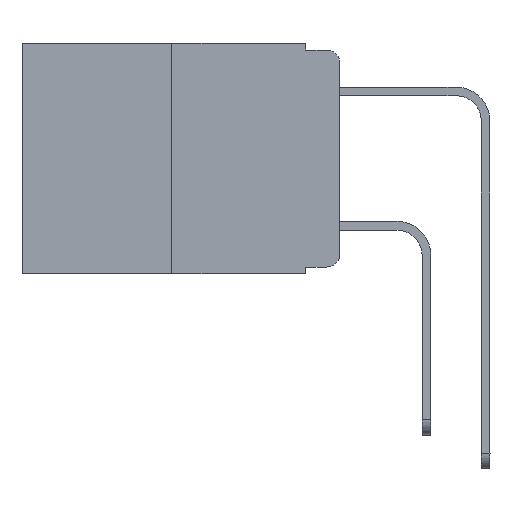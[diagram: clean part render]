
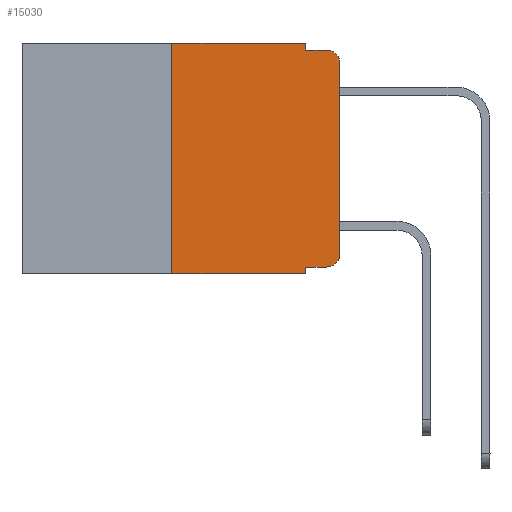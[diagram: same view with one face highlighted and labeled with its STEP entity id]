
A CAD part, left-side view. The second image highlights one B-rep face of the part: STEP entity #15030.
In plain terms, the highlighted planar face has unit normal (-1, 0, 0).
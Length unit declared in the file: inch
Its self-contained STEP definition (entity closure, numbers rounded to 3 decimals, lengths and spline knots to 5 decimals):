
#207 = EDGE_CURVE ( 'NONE', #6247, #10299, #6073, .T. ) ;
#486 = CARTESIAN_POINT ( 'NONE',  ( 0., 0., -0.313 ) ) ;
#516 = ORIENTED_EDGE ( 'NONE', *, *, #3117, .F. ) ;
#582 = CARTESIAN_POINT ( 'NONE',  ( 0., 0.02, -0.03 ) ) ;
#594 = CARTESIAN_POINT ( 'NONE',  ( 0., 0.051, 0. ) ) ;
#1008 = CARTESIAN_POINT ( 'NONE',  ( 0., 0.051, -0.01 ) ) ;
#1221 = VECTOR ( 'NONE', #10466, 39.37008 ) ;
#1612 = DIRECTION ( 'NONE',  ( 0., 0., -1. ) ) ;
#1639 = VERTEX_POINT ( 'NONE', #12210 ) ;
#1788 = EDGE_CURVE ( 'NONE', #15537, #11112, #16795, .T. ) ;
#2169 = CARTESIAN_POINT ( 'NONE',  ( 0., 0.473, 0. ) ) ;
#2224 = EDGE_CURVE ( 'NONE', #1639, #7217, #5862, .T. ) ;
#2312 = ORIENTED_EDGE ( 'NONE', *, *, #7118, .T. ) ;
#2544 = CIRCLE ( 'NONE', #13064, 0.02 ) ;
#2731 = PLANE ( 'NONE',  #8176 ) ;
#2915 = EDGE_CURVE ( 'NONE', #8779, #1639, #10983, .T. ) ;
#3005 = EDGE_CURVE ( 'NONE', #9134, #11112, #12538, .T. ) ;
#3117 = EDGE_CURVE ( 'NONE', #9134, #13423, #5496, .T. ) ;
#3352 = ORIENTED_EDGE ( 'NONE', *, *, #207, .T. ) ;
#3927 = CARTESIAN_POINT ( 'NONE',  ( 0., 0., 0. ) ) ;
#4178 = CARTESIAN_POINT ( 'NONE',  ( 0., 0.25, 0. ) ) ;
#4199 = ORIENTED_EDGE ( 'NONE', *, *, #1788, .F. ) ;
#4549 = CARTESIAN_POINT ( 'NONE',  ( 0., 0.02, -0.01 ) ) ;
#4834 = CARTESIAN_POINT ( 'NONE',  ( 0., 0.02, -0.333 ) ) ;
#4886 = CARTESIAN_POINT ( 'NONE',  ( 0., 0.051, -0.333 ) ) ;
#4983 = CARTESIAN_POINT ( 'NONE',  ( 0., 0.25, -0.343 ) ) ;
#5496 = LINE ( 'NONE', #11074, #15438 ) ;
#5862 = LINE ( 'NONE', #1008, #12071 ) ;
#6073 = CIRCLE ( 'NONE', #12502, 0.02 ) ;
#6105 = VERTEX_POINT ( 'NONE', #12702 ) ;
#6191 = ORIENTED_EDGE ( 'NONE', *, *, #12953, .T. ) ;
#6247 = VERTEX_POINT ( 'NONE', #4834 ) ;
#6763 = CARTESIAN_POINT ( 'NONE',  ( 0., 0.473, 0. ) ) ;
#6958 = DIRECTION ( 'NONE',  ( 0., -1., 0. ) ) ;
#7028 = CARTESIAN_POINT ( 'NONE',  ( 0., 0.051, -0.343 ) ) ;
#7118 = EDGE_CURVE ( 'NONE', #10299, #6105, #13632, .T. ) ;
#7217 = VERTEX_POINT ( 'NONE', #4549 ) ;
#7561 = LINE ( 'NONE', #2169, #12406 ) ;
#8142 = CARTESIAN_POINT ( 'NONE',  ( 0., 0.051, 0. ) ) ;
#8168 = CARTESIAN_POINT ( 'NONE',  ( 0., 0.051, 0. ) ) ;
#8176 = AXIS2_PLACEMENT_3D ( 'NONE', #6763, #15371, #11148 ) ;
#8281 = DIRECTION ( 'NONE',  ( -1., 0., 0. ) ) ;
#8538 = VECTOR ( 'NONE', #12185, 39.37008 ) ;
#8729 = EDGE_CURVE ( 'NONE', #13423, #8779, #7561, .T. ) ;
#8779 = VERTEX_POINT ( 'NONE', #594 ) ;
#8935 = ORIENTED_EDGE ( 'NONE', *, *, #8729, .F. ) ;
#9134 = VERTEX_POINT ( 'NONE', #4983 ) ;
#9654 = CARTESIAN_POINT ( 'NONE',  ( 0., 0.02, -0.313 ) ) ;
#9704 = VECTOR ( 'NONE', #6958, 39.37008 ) ;
#10299 = VERTEX_POINT ( 'NONE', #486 ) ;
#10466 = DIRECTION ( 'NONE',  ( 0., -1., 0. ) ) ;
#10656 = EDGE_LOOP ( 'NONE', ( #2312, #6191, #13620, #11908, #8935, #516, #12462, #4199, #15933, #3352 ) ) ;
#10967 = FACE_OUTER_BOUND ( 'NONE', #10656, .T. ) ;
#10983 = LINE ( 'NONE', #8142, #8538 ) ;
#11074 = CARTESIAN_POINT ( 'NONE',  ( 0., 0.25, 0. ) ) ;
#11076 = DIRECTION ( 'NONE',  ( 0., -1., 0. ) ) ;
#11112 = VERTEX_POINT ( 'NONE', #7028 ) ;
#11148 = DIRECTION ( 'NONE',  ( 0., 0., -1. ) ) ;
#11908 = ORIENTED_EDGE ( 'NONE', *, *, #2915, .F. ) ;
#12071 = VECTOR ( 'NONE', #11076, 39.37008 ) ;
#12185 = DIRECTION ( 'NONE',  ( 0., 0., -1. ) ) ;
#12210 = CARTESIAN_POINT ( 'NONE',  ( 0., 0.051, -0.01 ) ) ;
#12406 = VECTOR ( 'NONE', #17670, 39.37008 ) ;
#12462 = ORIENTED_EDGE ( 'NONE', *, *, #3005, .T. ) ;
#12502 = AXIS2_PLACEMENT_3D ( 'NONE', #9654, #8281, #16456 ) ;
#12538 = LINE ( 'NONE', #15482, #9704 ) ;
#12702 = CARTESIAN_POINT ( 'NONE',  ( 0., 0., -0.03 ) ) ;
#12953 = EDGE_CURVE ( 'NONE', #6105, #7217, #2544, .T. ) ;
#13064 = AXIS2_PLACEMENT_3D ( 'NONE', #582, #15723, #1612 ) ;
#13399 = LINE ( 'NONE', #4886, #1221 ) ;
#13423 = VERTEX_POINT ( 'NONE', #4178 ) ;
#13620 = ORIENTED_EDGE ( 'NONE', *, *, #2224, .F. ) ;
#13632 = LINE ( 'NONE', #3927, #17075 ) ;
#13886 = CARTESIAN_POINT ( 'NONE',  ( 0., 0.051, -0.333 ) ) ;
#14972 = EDGE_CURVE ( 'NONE', #15537, #6247, #13399, .T. ) ;
#15004 = DIRECTION ( 'NONE',  ( 0., 0., 1. ) ) ;
#15030 = ADVANCED_FACE ( 'NONE', ( #10967 ), #2731, .F. ) ;
#15315 = DIRECTION ( 'NONE',  ( 0., 0., -1. ) ) ;
#15371 = DIRECTION ( 'NONE',  ( 1., 0., 0. ) ) ;
#15438 = VECTOR ( 'NONE', #17570, 39.37008 ) ;
#15482 = CARTESIAN_POINT ( 'NONE',  ( 0., 0.473, -0.343 ) ) ;
#15537 = VERTEX_POINT ( 'NONE', #13886 ) ;
#15723 = DIRECTION ( 'NONE',  ( -1., 0., 0. ) ) ;
#15933 = ORIENTED_EDGE ( 'NONE', *, *, #14972, .T. ) ;
#16456 = DIRECTION ( 'NONE',  ( 0., 0., -1. ) ) ;
#16754 = VECTOR ( 'NONE', #15315, 39.37008 ) ;
#16795 = LINE ( 'NONE', #8168, #16754 ) ;
#17075 = VECTOR ( 'NONE', #15004, 39.37008 ) ;
#17570 = DIRECTION ( 'NONE',  ( 0., 0., 1. ) ) ;
#17670 = DIRECTION ( 'NONE',  ( 0., -1., 0. ) ) ;
